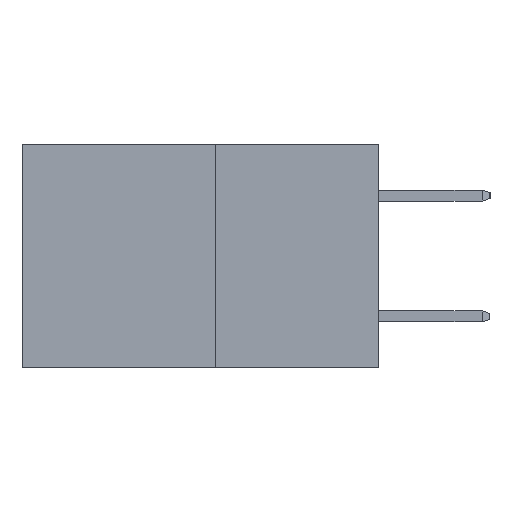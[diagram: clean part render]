
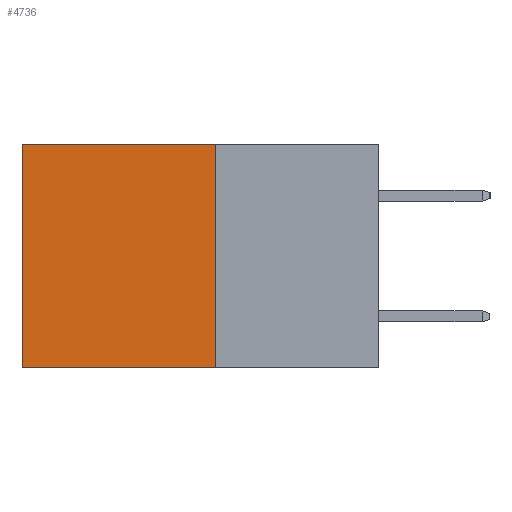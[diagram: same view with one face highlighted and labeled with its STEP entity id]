
A CAD part, left-side view. The second image highlights one B-rep face of the part: STEP entity #4736.
In plain terms, the highlighted planar face has unit normal (-1, 0, 0).
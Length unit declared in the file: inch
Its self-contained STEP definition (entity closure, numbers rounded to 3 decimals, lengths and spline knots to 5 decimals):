
#158 = LINE ( 'NONE', #9811, #3648 ) ;
#271 = CARTESIAN_POINT ( 'NONE',  ( 0.277, 0.59, -0.37 ) ) ;
#449 = DIRECTION ( 'NONE',  ( 0., 0., -1. ) ) ;
#527 = CARTESIAN_POINT ( 'NONE',  ( 0.277, 0.27, -0.37 ) ) ;
#1638 = VECTOR ( 'NONE', #1872, 39.37008 ) ;
#1872 = DIRECTION ( 'NONE',  ( 0., 1., 0. ) ) ;
#2108 = VERTEX_POINT ( 'NONE', #9863 ) ;
#2396 = VECTOR ( 'NONE', #449, 39.37008 ) ;
#2483 = EDGE_LOOP ( 'NONE', ( #15317, #15788, #9526, #6257 ) ) ;
#2878 = VERTEX_POINT ( 'NONE', #11637 ) ;
#3162 = VERTEX_POINT ( 'NONE', #3695 ) ;
#3281 = CARTESIAN_POINT ( 'NONE',  ( 0.277, 0.27, -0.37 ) ) ;
#3486 = EDGE_CURVE ( 'NONE', #2878, #9077, #14793, .T. ) ;
#3648 = VECTOR ( 'NONE', #9797, 39.37008 ) ;
#3695 = CARTESIAN_POINT ( 'NONE',  ( 0.277, 0.27, 0. ) ) ;
#4094 = EDGE_CURVE ( 'NONE', #3162, #2878, #7402, .T. ) ;
#4190 = DIRECTION ( 'NONE',  ( 0., 0., -1. ) ) ;
#4736 = ADVANCED_FACE ( 'NONE', ( #9487 ), #5191, .F. ) ;
#5191 = PLANE ( 'NONE',  #10434 ) ;
#6257 = ORIENTED_EDGE ( 'NONE', *, *, #6878, .T. ) ;
#6574 = EDGE_CURVE ( 'NONE', #2108, #9077, #15033, .T. ) ;
#6878 = EDGE_CURVE ( 'NONE', #3162, #2108, #158, .T. ) ;
#7402 = LINE ( 'NONE', #3281, #10269 ) ;
#7937 = DIRECTION ( 'NONE',  ( 0., 0., -1. ) ) ;
#9058 = DIRECTION ( 'NONE',  ( 1., 0., 0. ) ) ;
#9077 = VERTEX_POINT ( 'NONE', #10265 ) ;
#9154 = CARTESIAN_POINT ( 'NONE',  ( 0.277, 0.27, -0.37 ) ) ;
#9487 = FACE_OUTER_BOUND ( 'NONE', #2483, .T. ) ;
#9526 = ORIENTED_EDGE ( 'NONE', *, *, #4094, .F. ) ;
#9797 = DIRECTION ( 'NONE',  ( 0., 1., 0. ) ) ;
#9811 = CARTESIAN_POINT ( 'NONE',  ( 0.277, 0.27, 0. ) ) ;
#9863 = CARTESIAN_POINT ( 'NONE',  ( 0.277, 0.59, 0. ) ) ;
#10265 = CARTESIAN_POINT ( 'NONE',  ( 0.277, 0.59, -0.37 ) ) ;
#10269 = VECTOR ( 'NONE', #4190, 39.37008 ) ;
#10434 = AXIS2_PLACEMENT_3D ( 'NONE', #9154, #9058, #7937 ) ;
#11637 = CARTESIAN_POINT ( 'NONE',  ( 0.277, 0.27, -0.37 ) ) ;
#14793 = LINE ( 'NONE', #527, #1638 ) ;
#15033 = LINE ( 'NONE', #271, #2396 ) ;
#15317 = ORIENTED_EDGE ( 'NONE', *, *, #6574, .T. ) ;
#15788 = ORIENTED_EDGE ( 'NONE', *, *, #3486, .F. ) ;
